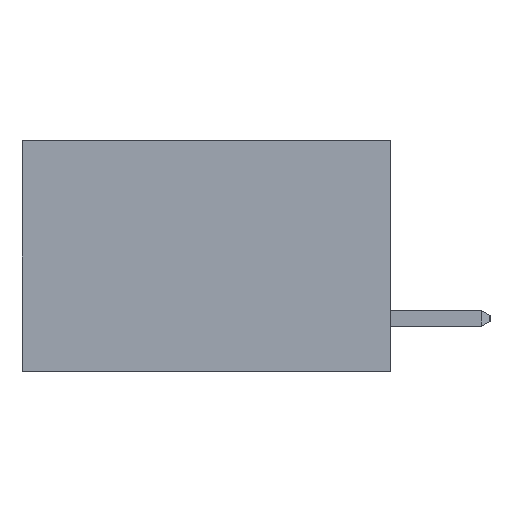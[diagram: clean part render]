
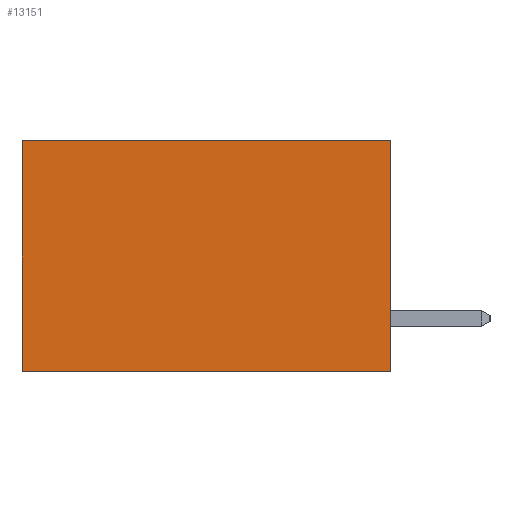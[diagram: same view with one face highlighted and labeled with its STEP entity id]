
A CAD part, left-side view. The second image highlights one B-rep face of the part: STEP entity #13151.
In plain terms, the highlighted planar face has unit normal (-1, 0, 0).
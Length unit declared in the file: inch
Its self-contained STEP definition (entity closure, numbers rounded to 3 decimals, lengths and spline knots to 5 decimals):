
#155 = LINE ( 'NONE', #691, #11014 ) ;
#691 = CARTESIAN_POINT ( 'NONE',  ( 0.277, 0., -0.37 ) ) ;
#735 = CARTESIAN_POINT ( 'NONE',  ( 0.277, 0., 0. ) ) ;
#1147 = EDGE_LOOP ( 'NONE', ( #2507, #2576, #2763, #2868 ) ) ;
#1486 = CARTESIAN_POINT ( 'NONE',  ( 0.277, 0., 0. ) ) ;
#1856 = VERTEX_POINT ( 'NONE', #735 ) ;
#1966 = DIRECTION ( 'NONE',  ( 0., 0., -1. ) ) ;
#2507 = ORIENTED_EDGE ( 'NONE', *, *, #2949, .T. ) ;
#2576 = ORIENTED_EDGE ( 'NONE', *, *, #5985, .F. ) ;
#2681 = VECTOR ( 'NONE', #10678, 39.37008 ) ;
#2763 = ORIENTED_EDGE ( 'NONE', *, *, #9026, .F. ) ;
#2868 = ORIENTED_EDGE ( 'NONE', *, *, #11063, .T. ) ;
#2949 = EDGE_CURVE ( 'NONE', #11387, #6379, #14596, .T. ) ;
#4281 = CARTESIAN_POINT ( 'NONE',  ( 0.277, 0., -0.37 ) ) ;
#4498 = CARTESIAN_POINT ( 'NONE',  ( 0.277, 0.59, -0.37 ) ) ;
#5254 = VECTOR ( 'NONE', #13984, 39.37008 ) ;
#5413 = PLANE ( 'NONE',  #13643 ) ;
#5470 = DIRECTION ( 'NONE',  ( 0., 0., -1. ) ) ;
#5985 = EDGE_CURVE ( 'NONE', #10531, #6379, #11182, .T. ) ;
#6379 = VERTEX_POINT ( 'NONE', #8047 ) ;
#8047 = CARTESIAN_POINT ( 'NONE',  ( 0.277, 0.59, -0.37 ) ) ;
#8405 = LINE ( 'NONE', #1486, #2681 ) ;
#9026 = EDGE_CURVE ( 'NONE', #1856, #10531, #155, .T. ) ;
#9176 = CARTESIAN_POINT ( 'NONE',  ( 0.277, 0., -0.37 ) ) ;
#10531 = VERTEX_POINT ( 'NONE', #9176 ) ;
#10678 = DIRECTION ( 'NONE',  ( 0., 1., 0. ) ) ;
#11014 = VECTOR ( 'NONE', #1966, 39.37008 ) ;
#11063 = EDGE_CURVE ( 'NONE', #1856, #11387, #8405, .T. ) ;
#11141 = CARTESIAN_POINT ( 'NONE',  ( 0.277, 0.59, 0. ) ) ;
#11182 = LINE ( 'NONE', #14053, #5254 ) ;
#11387 = VERTEX_POINT ( 'NONE', #11141 ) ;
#11421 = VECTOR ( 'NONE', #11548, 39.37008 ) ;
#11548 = DIRECTION ( 'NONE',  ( 0., 0., -1. ) ) ;
#12110 = DIRECTION ( 'NONE',  ( 1., 0., 0. ) ) ;
#13151 = ADVANCED_FACE ( 'NONE', ( #14126 ), #5413, .F. ) ;
#13643 = AXIS2_PLACEMENT_3D ( 'NONE', #4281, #12110, #5470 ) ;
#13984 = DIRECTION ( 'NONE',  ( 0., 1., 0. ) ) ;
#14053 = CARTESIAN_POINT ( 'NONE',  ( 0.277, 0., -0.37 ) ) ;
#14126 = FACE_OUTER_BOUND ( 'NONE', #1147, .T. ) ;
#14596 = LINE ( 'NONE', #4498, #11421 ) ;
